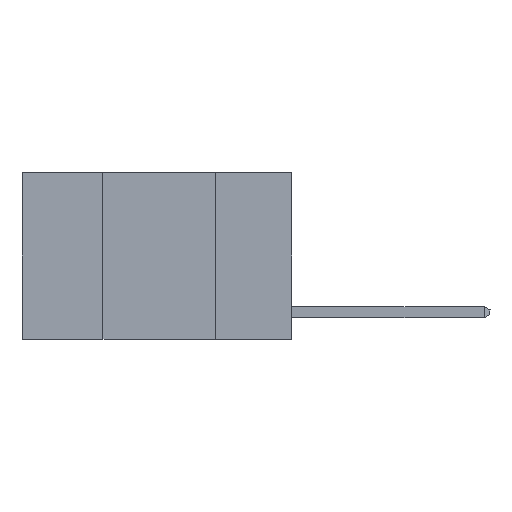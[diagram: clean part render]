
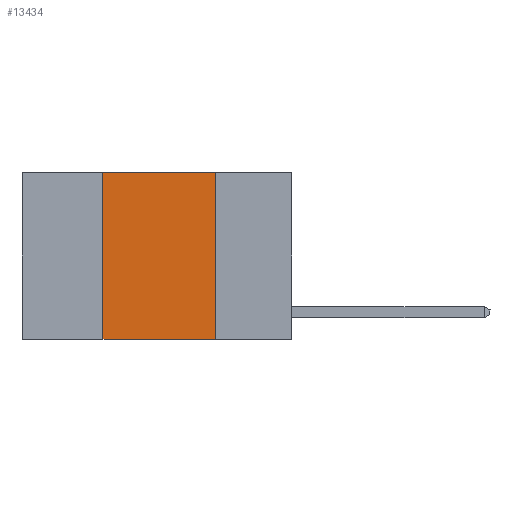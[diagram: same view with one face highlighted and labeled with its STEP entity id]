
A CAD part, left-side view. The second image highlights one B-rep face of the part: STEP entity #13434.
In plain terms, the highlighted planar face has unit normal (-1, 0, 0).
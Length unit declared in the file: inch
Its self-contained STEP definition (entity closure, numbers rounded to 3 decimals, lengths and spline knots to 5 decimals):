
#90 = LINE ( 'NONE', #10362, #20377 ) ;
#841 = EDGE_CURVE ( 'NONE', #8299, #5459, #21175, .T. ) ;
#866 = ORIENTED_EDGE ( 'NONE', *, *, #6078, .F. ) ;
#1550 = VECTOR ( 'NONE', #7232, 39.37008 ) ;
#2417 = EDGE_CURVE ( 'NONE', #18009, #8299, #13396, .T. ) ;
#3759 = VECTOR ( 'NONE', #21945, 39.37008 ) ;
#3889 = CARTESIAN_POINT ( 'NONE',  ( 0., 0.17, -0.37 ) ) ;
#4104 = CARTESIAN_POINT ( 'NONE',  ( 0., 0.6, 0. ) ) ;
#5459 = VERTEX_POINT ( 'NONE', #22793 ) ;
#5920 = DIRECTION ( 'NONE',  ( 0., 0., -1. ) ) ;
#6078 = EDGE_CURVE ( 'NONE', #5459, #8474, #90, .T. ) ;
#7232 = DIRECTION ( 'NONE',  ( 0., -1., 0. ) ) ;
#8299 = VERTEX_POINT ( 'NONE', #17862 ) ;
#8429 = FACE_OUTER_BOUND ( 'NONE', #23026, .T. ) ;
#8474 = VERTEX_POINT ( 'NONE', #3889 ) ;
#8878 = ORIENTED_EDGE ( 'NONE', *, *, #22079, .T. ) ;
#9276 = ORIENTED_EDGE ( 'NONE', *, *, #841, .F. ) ;
#10362 = CARTESIAN_POINT ( 'NONE',  ( 0., 0.17, 0. ) ) ;
#11096 = ORIENTED_EDGE ( 'NONE', *, *, #2417, .F. ) ;
#13396 = LINE ( 'NONE', #21927, #3759 ) ;
#13434 = ADVANCED_FACE ( 'NONE', ( #8429 ), #21921, .F. ) ;
#15722 = DIRECTION ( 'NONE',  ( 0., 0., -1. ) ) ;
#15926 = AXIS2_PLACEMENT_3D ( 'NONE', #4104, #16751, #5920 ) ;
#16751 = DIRECTION ( 'NONE',  ( 1., 0., 0. ) ) ;
#17255 = LINE ( 'NONE', #20811, #21295 ) ;
#17862 = CARTESIAN_POINT ( 'NONE',  ( 0., 0.42, 0. ) ) ;
#18009 = VERTEX_POINT ( 'NONE', #19042 ) ;
#19042 = CARTESIAN_POINT ( 'NONE',  ( 0., 0.42, -0.37 ) ) ;
#19116 = CARTESIAN_POINT ( 'NONE',  ( 0., 0.6, 0. ) ) ;
#20377 = VECTOR ( 'NONE', #15722, 39.37008 ) ;
#20811 = CARTESIAN_POINT ( 'NONE',  ( 0., 0.6, -0.37 ) ) ;
#21175 = LINE ( 'NONE', #19116, #1550 ) ;
#21295 = VECTOR ( 'NONE', #22617, 39.37008 ) ;
#21921 = PLANE ( 'NONE',  #15926 ) ;
#21927 = CARTESIAN_POINT ( 'NONE',  ( 0., 0.42, 0. ) ) ;
#21945 = DIRECTION ( 'NONE',  ( 0., 0., 1. ) ) ;
#22079 = EDGE_CURVE ( 'NONE', #18009, #8474, #17255, .T. ) ;
#22617 = DIRECTION ( 'NONE',  ( 0., -1., 0. ) ) ;
#22793 = CARTESIAN_POINT ( 'NONE',  ( 0., 0.17, 0. ) ) ;
#23026 = EDGE_LOOP ( 'NONE', ( #866, #9276, #11096, #8878 ) ) ;
